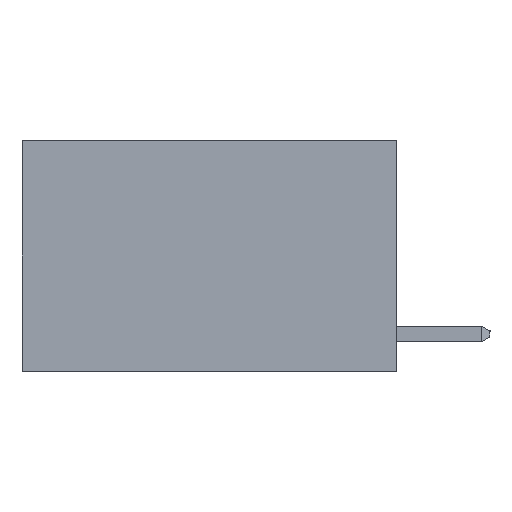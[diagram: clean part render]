
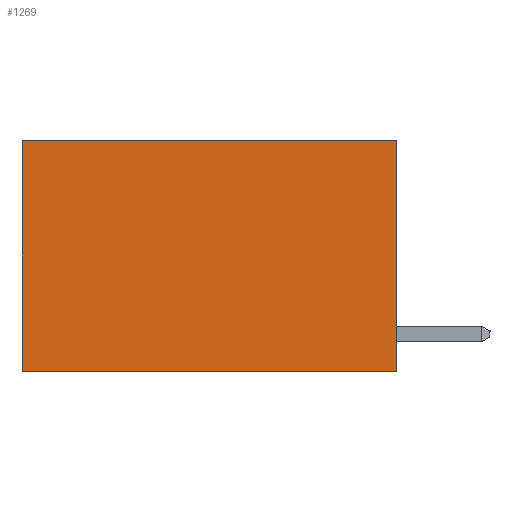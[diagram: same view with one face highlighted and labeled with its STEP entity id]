
A CAD part, left-side view. The second image highlights one B-rep face of the part: STEP entity #1269.
In plain terms, the highlighted planar face has unit normal (-1, 0, 0).
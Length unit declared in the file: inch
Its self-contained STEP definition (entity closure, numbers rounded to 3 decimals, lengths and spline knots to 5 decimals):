
#339 = FACE_OUTER_BOUND ( 'NONE', #7347, .T. ) ;
#967 = CARTESIAN_POINT ( 'NONE',  ( 0.2625, 0., -0.37 ) ) ;
#1269 = ADVANCED_FACE ( 'NONE', ( #339 ), #15228, .F. ) ;
#1331 = DIRECTION ( 'NONE',  ( 0., 0., -1. ) ) ;
#1954 = VERTEX_POINT ( 'NONE', #9316 ) ;
#2925 = ORIENTED_EDGE ( 'NONE', *, *, #9357, .T. ) ;
#3770 = DIRECTION ( 'NONE',  ( 0., 1., 0. ) ) ;
#3798 = DIRECTION ( 'NONE',  ( 0., 0., -1. ) ) ;
#4653 = ORIENTED_EDGE ( 'NONE', *, *, #14131, .T. ) ;
#4925 = AXIS2_PLACEMENT_3D ( 'NONE', #11843, #6105, #13045 ) ;
#5325 = VECTOR ( 'NONE', #3798, 39.37008 ) ;
#5812 = VERTEX_POINT ( 'NONE', #9080 ) ;
#6105 = DIRECTION ( 'NONE',  ( 1., 0., 0. ) ) ;
#7347 = EDGE_LOOP ( 'NONE', ( #2925, #12061, #13785, #4653 ) ) ;
#7371 = VERTEX_POINT ( 'NONE', #10068 ) ;
#7928 = EDGE_CURVE ( 'NONE', #1954, #11922, #12986, .T. ) ;
#7958 = VECTOR ( 'NONE', #3770, 39.37008 ) ;
#8658 = LINE ( 'NONE', #10100, #5325 ) ;
#9080 = CARTESIAN_POINT ( 'NONE',  ( 0.2625, 0., 0. ) ) ;
#9316 = CARTESIAN_POINT ( 'NONE',  ( 0.2625, 0., -0.37 ) ) ;
#9357 = EDGE_CURVE ( 'NONE', #7371, #11922, #15328, .T. ) ;
#9504 = CARTESIAN_POINT ( 'NONE',  ( 0.2625, 0.6, -0.37 ) ) ;
#10068 = CARTESIAN_POINT ( 'NONE',  ( 0.2625, 0.6, 0. ) ) ;
#10100 = CARTESIAN_POINT ( 'NONE',  ( 0.2625, 0., 0. ) ) ;
#11246 = DIRECTION ( 'NONE',  ( 0., 1., 0. ) ) ;
#11574 = VECTOR ( 'NONE', #1331, 39.37008 ) ;
#11843 = CARTESIAN_POINT ( 'NONE',  ( 0.2625, 0., 0. ) ) ;
#11922 = VERTEX_POINT ( 'NONE', #9504 ) ;
#12061 = ORIENTED_EDGE ( 'NONE', *, *, #7928, .F. ) ;
#12581 = CARTESIAN_POINT ( 'NONE',  ( 0.2625, 0., 0. ) ) ;
#12598 = VECTOR ( 'NONE', #11246, 39.37008 ) ;
#12986 = LINE ( 'NONE', #967, #12598 ) ;
#13045 = DIRECTION ( 'NONE',  ( 0., 0., -1. ) ) ;
#13785 = ORIENTED_EDGE ( 'NONE', *, *, #15827, .F. ) ;
#14131 = EDGE_CURVE ( 'NONE', #5812, #7371, #14602, .T. ) ;
#14602 = LINE ( 'NONE', #12581, #7958 ) ;
#15228 = PLANE ( 'NONE',  #4925 ) ;
#15328 = LINE ( 'NONE', #16306, #11574 ) ;
#15827 = EDGE_CURVE ( 'NONE', #5812, #1954, #8658, .T. ) ;
#16306 = CARTESIAN_POINT ( 'NONE',  ( 0.2625, 0.6, 0. ) ) ;
